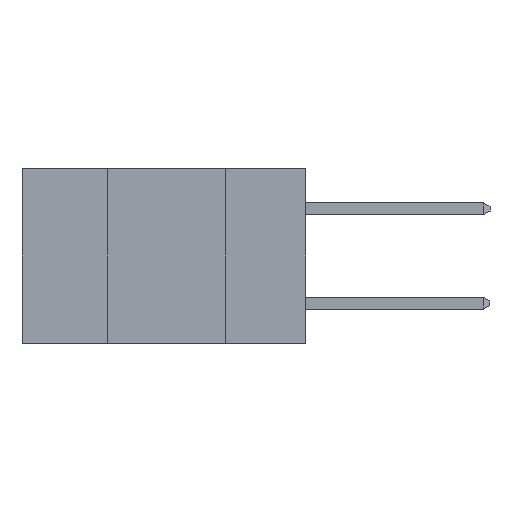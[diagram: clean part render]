
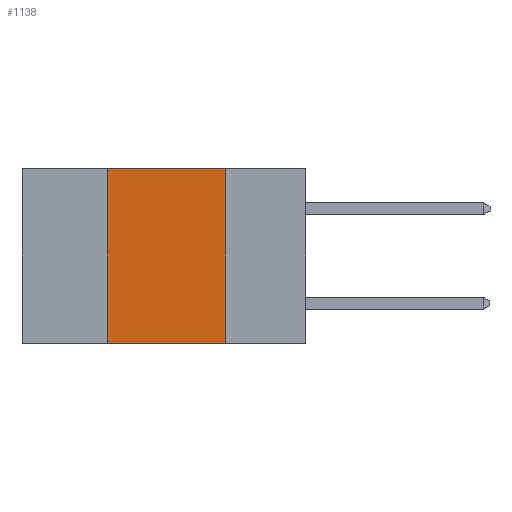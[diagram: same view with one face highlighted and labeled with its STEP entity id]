
A CAD part, left-side view. The second image highlights one B-rep face of the part: STEP entity #1138.
In plain terms, the highlighted planar face has unit normal (-1, 0, 0).
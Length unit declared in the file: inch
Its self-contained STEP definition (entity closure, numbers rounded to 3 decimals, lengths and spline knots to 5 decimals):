
#292 = CARTESIAN_POINT ( 'NONE',  ( 0., 0.42, 0. ) ) ;
#380 = CARTESIAN_POINT ( 'NONE',  ( 0., 0.6, 0. ) ) ;
#505 = EDGE_LOOP ( 'NONE', ( #19127, #13582, #17938, #13211 ) ) ;
#1138 = ADVANCED_FACE ( 'NONE', ( #13778 ), #4924, .F. ) ;
#1151 = DIRECTION ( 'NONE',  ( 0., -1., 0. ) ) ;
#1694 = DIRECTION ( 'NONE',  ( 0., 0., -1. ) ) ;
#1820 = VERTEX_POINT ( 'NONE', #3960 ) ;
#2400 = CARTESIAN_POINT ( 'NONE',  ( 0., 0.42, -0.37 ) ) ;
#2563 = AXIS2_PLACEMENT_3D ( 'NONE', #380, #13335, #10980 ) ;
#2907 = CARTESIAN_POINT ( 'NONE',  ( 0., 0.42, 0. ) ) ;
#3960 = CARTESIAN_POINT ( 'NONE',  ( 0., 0.17, -0.37 ) ) ;
#4487 = DIRECTION ( 'NONE',  ( 0., 0., 1. ) ) ;
#4592 = LINE ( 'NONE', #12732, #8251 ) ;
#4917 = LINE ( 'NONE', #12730, #18009 ) ;
#4924 = PLANE ( 'NONE',  #2563 ) ;
#5006 = VECTOR ( 'NONE', #1151, 39.37008 ) ;
#5843 = CARTESIAN_POINT ( 'NONE',  ( 0., 0.6, 0. ) ) ;
#6029 = VERTEX_POINT ( 'NONE', #2400 ) ;
#8251 = VECTOR ( 'NONE', #1694, 39.37008 ) ;
#8854 = VERTEX_POINT ( 'NONE', #292 ) ;
#9209 = EDGE_CURVE ( 'NONE', #8854, #11587, #13469, .T. ) ;
#10679 = EDGE_CURVE ( 'NONE', #6029, #8854, #15079, .T. ) ;
#10980 = DIRECTION ( 'NONE',  ( 0., 0., -1. ) ) ;
#11587 = VERTEX_POINT ( 'NONE', #12412 ) ;
#12412 = CARTESIAN_POINT ( 'NONE',  ( 0., 0.17, 0. ) ) ;
#12730 = CARTESIAN_POINT ( 'NONE',  ( 0., 0.6, -0.37 ) ) ;
#12732 = CARTESIAN_POINT ( 'NONE',  ( 0., 0.17, 0. ) ) ;
#13211 = ORIENTED_EDGE ( 'NONE', *, *, #18212, .T. ) ;
#13335 = DIRECTION ( 'NONE',  ( 1., 0., 0. ) ) ;
#13469 = LINE ( 'NONE', #5843, #5006 ) ;
#13582 = ORIENTED_EDGE ( 'NONE', *, *, #9209, .F. ) ;
#13778 = FACE_OUTER_BOUND ( 'NONE', #505, .T. ) ;
#15079 = LINE ( 'NONE', #2907, #19140 ) ;
#17938 = ORIENTED_EDGE ( 'NONE', *, *, #10679, .F. ) ;
#18009 = VECTOR ( 'NONE', #18918, 39.37008 ) ;
#18212 = EDGE_CURVE ( 'NONE', #6029, #1820, #4917, .T. ) ;
#18918 = DIRECTION ( 'NONE',  ( 0., -1., 0. ) ) ;
#19127 = ORIENTED_EDGE ( 'NONE', *, *, #20089, .F. ) ;
#19140 = VECTOR ( 'NONE', #4487, 39.37008 ) ;
#20089 = EDGE_CURVE ( 'NONE', #11587, #1820, #4592, .T. ) ;
